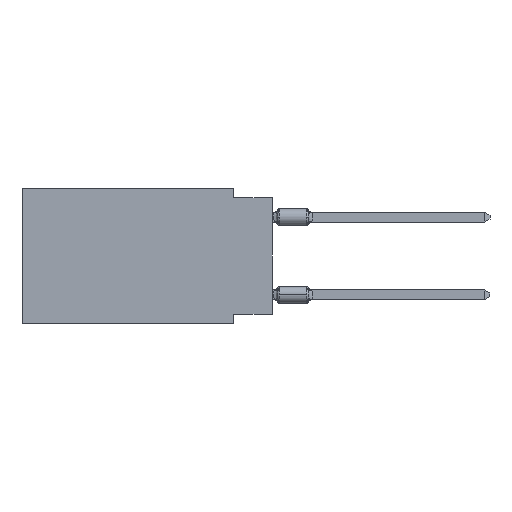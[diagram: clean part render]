
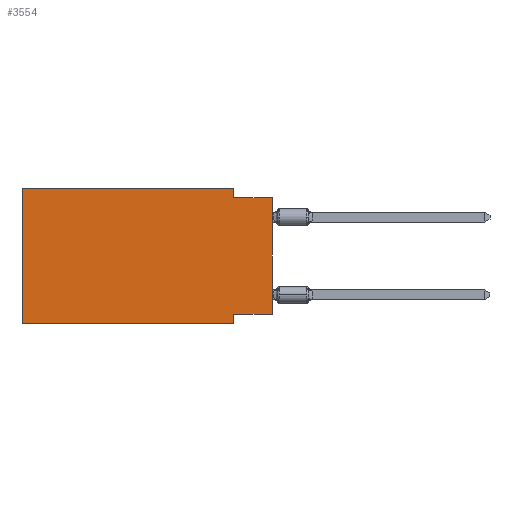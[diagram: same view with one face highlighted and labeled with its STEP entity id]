
A CAD part, left-side view. The second image highlights one B-rep face of the part: STEP entity #3554.
In plain terms, the highlighted planar face has unit normal (-1, 0, 0).
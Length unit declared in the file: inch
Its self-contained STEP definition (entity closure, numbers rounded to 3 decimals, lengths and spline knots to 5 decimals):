
#25 = CARTESIAN_POINT ( 'NONE',  ( 0., 0.645, -0.35 ) ) ;
#326 = LINE ( 'NONE', #2507, #16730 ) ;
#1002 = VECTOR ( 'NONE', #22798, 39.37008 ) ;
#1232 = EDGE_LOOP ( 'NONE', ( #19791, #9271, #20654, #6620, #16566, #15615, #19451, #1998 ) ) ;
#1248 = CARTESIAN_POINT ( 'NONE',  ( 0., 0.645, 0. ) ) ;
#1997 = CARTESIAN_POINT ( 'NONE',  ( 0., 0.645, 0. ) ) ;
#1998 = ORIENTED_EDGE ( 'NONE', *, *, #15115, .F. ) ;
#2501 = VECTOR ( 'NONE', #9557, 39.37008 ) ;
#2507 = CARTESIAN_POINT ( 'NONE',  ( 0., 0.645, 0. ) ) ;
#2853 = VECTOR ( 'NONE', #15311, 39.37008 ) ;
#3372 = PLANE ( 'NONE',  #4536 ) ;
#3489 = DIRECTION ( 'NONE',  ( 0., 0., -1. ) ) ;
#3554 = ADVANCED_FACE ( 'NONE', ( #12721 ), #3372, .F. ) ;
#3584 = DIRECTION ( 'NONE',  ( 0., 1., 0. ) ) ;
#3616 = CARTESIAN_POINT ( 'NONE',  ( 0., 0.1, -0.35 ) ) ;
#4355 = VECTOR ( 'NONE', #3584, 39.37008 ) ;
#4536 = AXIS2_PLACEMENT_3D ( 'NONE', #5241, #12371, #3489 ) ;
#4808 = VECTOR ( 'NONE', #13601, 39.37008 ) ;
#4816 = VERTEX_POINT ( 'NONE', #1997 ) ;
#5241 = CARTESIAN_POINT ( 'NONE',  ( 0., 0.645, 0. ) ) ;
#5440 = LINE ( 'NONE', #12222, #20404 ) ;
#6620 = ORIENTED_EDGE ( 'NONE', *, *, #20520, .F. ) ;
#6841 = CARTESIAN_POINT ( 'NONE',  ( 0., 0.1, 0. ) ) ;
#8694 = DIRECTION ( 'NONE',  ( 0., -1., 0. ) ) ;
#8822 = LINE ( 'NONE', #15980, #4355 ) ;
#9119 = VERTEX_POINT ( 'NONE', #25 ) ;
#9271 = ORIENTED_EDGE ( 'NONE', *, *, #16310, .F. ) ;
#9557 = DIRECTION ( 'NONE',  ( 0., 0., 1. ) ) ;
#9690 = CARTESIAN_POINT ( 'NONE',  ( 0., 0., -0.325 ) ) ;
#9741 = CARTESIAN_POINT ( 'NONE',  ( 0., 0.1, -0.025 ) ) ;
#10926 = CARTESIAN_POINT ( 'NONE',  ( 0., 0., -0.025 ) ) ;
#11029 = VERTEX_POINT ( 'NONE', #9690 ) ;
#11117 = VECTOR ( 'NONE', #13788, 39.37008 ) ;
#11614 = VERTEX_POINT ( 'NONE', #15419 ) ;
#12142 = LINE ( 'NONE', #3616, #1002 ) ;
#12222 = CARTESIAN_POINT ( 'NONE',  ( 0., 0., -0.025 ) ) ;
#12371 = DIRECTION ( 'NONE',  ( 1., 0., 0. ) ) ;
#12721 = FACE_OUTER_BOUND ( 'NONE', #1232, .T. ) ;
#12749 = VERTEX_POINT ( 'NONE', #6841 ) ;
#13025 = DIRECTION ( 'NONE',  ( 0., 0., 1. ) ) ;
#13601 = DIRECTION ( 'NONE',  ( 0., -1., 0. ) ) ;
#13788 = DIRECTION ( 'NONE',  ( 0., 0., -1. ) ) ;
#14150 = VERTEX_POINT ( 'NONE', #10926 ) ;
#14499 = VERTEX_POINT ( 'NONE', #15068 ) ;
#14554 = EDGE_CURVE ( 'NONE', #9119, #11614, #22195, .T. ) ;
#14705 = EDGE_CURVE ( 'NONE', #14499, #11614, #12142, .T. ) ;
#15068 = CARTESIAN_POINT ( 'NONE',  ( 0., 0.1, -0.325 ) ) ;
#15115 = EDGE_CURVE ( 'NONE', #11029, #14499, #8822, .T. ) ;
#15311 = DIRECTION ( 'NONE',  ( 0., -1., 0. ) ) ;
#15419 = CARTESIAN_POINT ( 'NONE',  ( 0., 0.1, -0.35 ) ) ;
#15615 = ORIENTED_EDGE ( 'NONE', *, *, #14554, .T. ) ;
#15980 = CARTESIAN_POINT ( 'NONE',  ( 0., 0., -0.325 ) ) ;
#16310 = EDGE_CURVE ( 'NONE', #21657, #14150, #5440, .T. ) ;
#16566 = ORIENTED_EDGE ( 'NONE', *, *, #17765, .F. ) ;
#16730 = VECTOR ( 'NONE', #13025, 39.37008 ) ;
#16837 = CARTESIAN_POINT ( 'NONE',  ( 0., 0.645, -0.35 ) ) ;
#16879 = EDGE_CURVE ( 'NONE', #11029, #14150, #20465, .T. ) ;
#17765 = EDGE_CURVE ( 'NONE', #9119, #4816, #326, .T. ) ;
#17926 = CARTESIAN_POINT ( 'NONE',  ( 0., 0., 0. ) ) ;
#19451 = ORIENTED_EDGE ( 'NONE', *, *, #14705, .F. ) ;
#19791 = ORIENTED_EDGE ( 'NONE', *, *, #16879, .T. ) ;
#19807 = EDGE_CURVE ( 'NONE', #12749, #21657, #22561, .T. ) ;
#20404 = VECTOR ( 'NONE', #8694, 39.37008 ) ;
#20465 = LINE ( 'NONE', #17926, #2501 ) ;
#20520 = EDGE_CURVE ( 'NONE', #4816, #12749, #20753, .T. ) ;
#20654 = ORIENTED_EDGE ( 'NONE', *, *, #19807, .F. ) ;
#20753 = LINE ( 'NONE', #1248, #4808 ) ;
#21657 = VERTEX_POINT ( 'NONE', #9741 ) ;
#22195 = LINE ( 'NONE', #16837, #2853 ) ;
#22561 = LINE ( 'NONE', #22922, #11117 ) ;
#22798 = DIRECTION ( 'NONE',  ( 0., 0., -1. ) ) ;
#22922 = CARTESIAN_POINT ( 'NONE',  ( 0., 0.1, 0. ) ) ;
